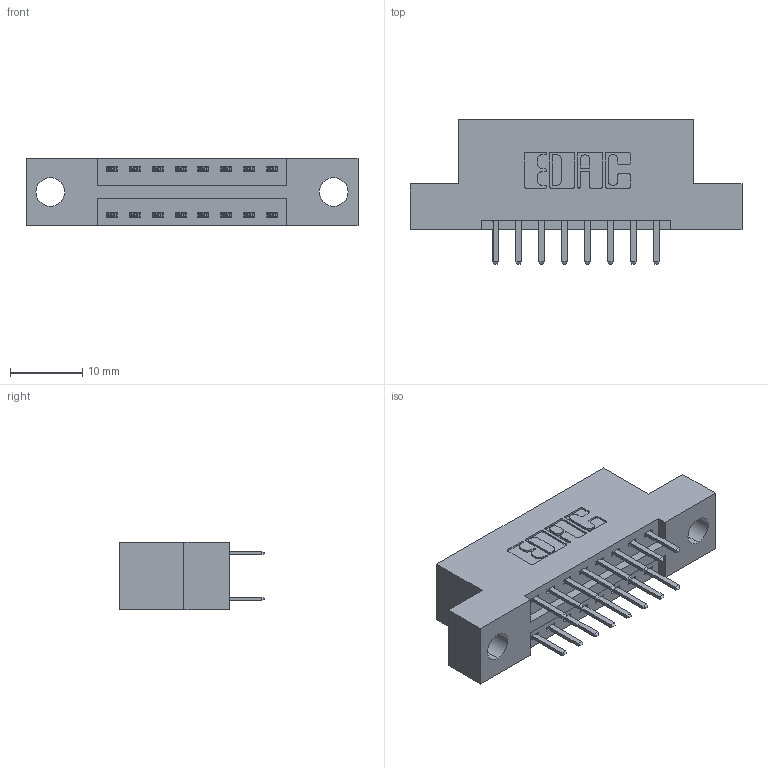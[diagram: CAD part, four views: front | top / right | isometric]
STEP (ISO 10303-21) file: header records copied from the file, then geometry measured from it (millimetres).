
FILE_DESCRIPTION (( 'STEP AP203' ), '1' );
FILE_NAME ('396-016-520-204.STEP', '2018-08-31T22:25:55', ( '' ), ( '' ), 'SwSTEP 2.0', 'SolidWorks 2016', '' );
FILE_SCHEMA (( 'CONFIG_CONTROL_DESIGN' ));
Length unit declared in the file: inch
Products named in the file (3): 346 Part_Flush Mounting Lugs - 0.156 Dia-TH; 345-292-001_345-293-120; 396-016-520-204
Assembly tree (17 placements, depth 2):
  396-016-520-204
    346 Part_Flush Mounting Lugs - 0.156 Dia-TH
    345-292-001_345-293-120  x16
Bounding box: 45.97 x 20.02 x 9.4 mm (x, y, z)
Volume: 4124.1 mm3; surface area: 4931.3 mm2
Topology: 17 solids, 17 shells, 1018 faces, 2937 edges, 1914 vertices
Faces by surface type: plane 668, cylinder 350
Entity records: 9915 total; most frequent: CARTESIAN_POINT 1692, ORIENTED_EDGE 1614, DIRECTION 1531, EDGE_CURVE 807, LINE 639, VECTOR 639, VERTEX_POINT 534, AXIS2_PLACEMENT_3D 446
